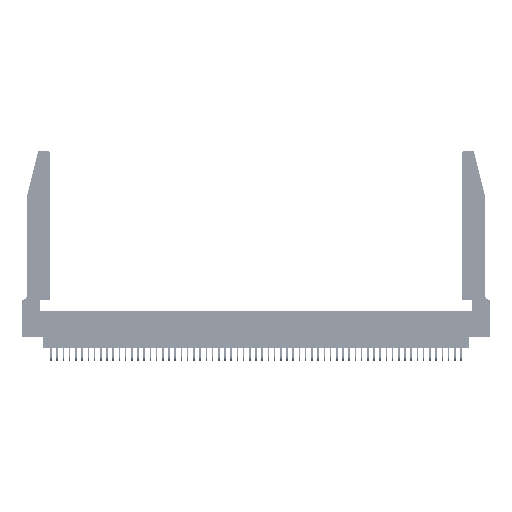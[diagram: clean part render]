
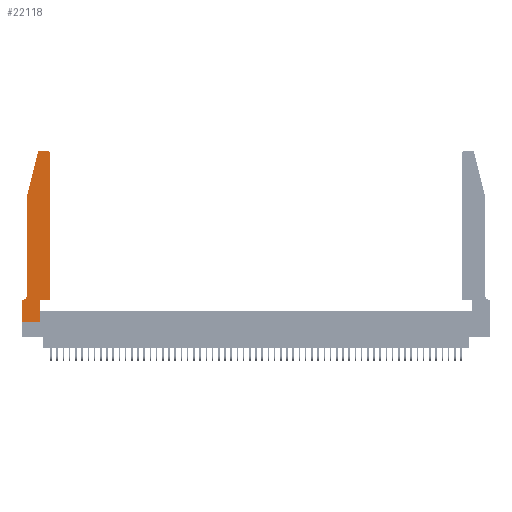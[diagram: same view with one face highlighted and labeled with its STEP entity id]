
A CAD part, top view. The second image highlights one B-rep face of the part: STEP entity #22118.
In plain terms, the highlighted planar face has unit normal (0, 0, 1).
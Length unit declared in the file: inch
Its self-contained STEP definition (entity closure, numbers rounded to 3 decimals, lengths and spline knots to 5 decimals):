
#448 = CIRCLE ( 'NONE', #9576, 0.03 ) ;
#577 = CARTESIAN_POINT ( 'NONE',  ( 0.4505, 0.35, 0.37 ) ) ;
#1251 = VERTEX_POINT ( 'NONE', #31348 ) ;
#1568 = LINE ( 'NONE', #27744, #34705 ) ;
#2363 = CARTESIAN_POINT ( 'NONE',  ( 0., 0.35, 0.37 ) ) ;
#2644 = ORIENTED_EDGE ( 'NONE', *, *, #7055, .T. ) ;
#3427 = VECTOR ( 'NONE', #39457, 39.37008 ) ;
#4058 = VERTEX_POINT ( 'NONE', #46979 ) ;
#4506 = VERTEX_POINT ( 'NONE', #54104 ) ;
#5450 = PLANE ( 'NONE',  #37151 ) ;
#6141 = DIRECTION ( 'NONE',  ( 0., -1., 0. ) ) ;
#7055 = EDGE_CURVE ( 'NONE', #8284, #24418, #36979, .T. ) ;
#7409 = LINE ( 'NONE', #52292, #51784 ) ;
#7909 = VERTEX_POINT ( 'NONE', #47162 ) ;
#8218 = CARTESIAN_POINT ( 'NONE',  ( 0.2865, 0.35, 0.37 ) ) ;
#8284 = VERTEX_POINT ( 'NONE', #2363 ) ;
#8522 = VERTEX_POINT ( 'NONE', #8218 ) ;
#9533 = ORIENTED_EDGE ( 'NONE', *, *, #33790, .T. ) ;
#9576 = AXIS2_PLACEMENT_3D ( 'NONE', #47927, #22349, #52252 ) ;
#9901 = DIRECTION ( 'NONE',  ( 0., 0., 1. ) ) ;
#10131 = ORIENTED_EDGE ( 'NONE', *, *, #50428, .T. ) ;
#10449 = VECTOR ( 'NONE', #50273, 39.37008 ) ;
#11404 = DIRECTION ( 'NONE',  ( 0., -1., 0. ) ) ;
#12452 = DIRECTION ( 'NONE',  ( -1., 0., 0. ) ) ;
#13493 = DIRECTION ( 'NONE',  ( 0., 0., -1. ) ) ;
#13606 = ORIENTED_EDGE ( 'NONE', *, *, #24213, .T. ) ;
#14256 = DIRECTION ( 'NONE',  ( 0., 0., 1. ) ) ;
#14684 = DIRECTION ( 'NONE',  ( 0., 1., 0. ) ) ;
#15362 = EDGE_CURVE ( 'NONE', #4506, #8284, #31526, .T. ) ;
#16904 = VECTOR ( 'NONE', #51063, 39.37008 ) ;
#18411 = CIRCLE ( 'NONE', #40693, 0.03 ) ;
#19035 = VERTEX_POINT ( 'NONE', #51246 ) ;
#19907 = EDGE_CURVE ( 'NONE', #24418, #42838, #7409, .T. ) ;
#20412 = VECTOR ( 'NONE', #41550, 39.37008 ) ;
#21118 = EDGE_CURVE ( 'NONE', #42838, #8522, #46048, .T. ) ;
#21649 = ORIENTED_EDGE ( 'NONE', *, *, #15362, .T. ) ;
#22118 = ADVANCED_FACE ( 'NONE', ( #40603 ), #5450, .T. ) ;
#22349 = DIRECTION ( 'NONE',  ( 0., 0., 1. ) ) ;
#22935 = EDGE_CURVE ( 'NONE', #7909, #19035, #44513, .T. ) ;
#24213 = EDGE_CURVE ( 'NONE', #54531, #1251, #48345, .T. ) ;
#24418 = VERTEX_POINT ( 'NONE', #31094 ) ;
#24508 = CARTESIAN_POINT ( 'NONE',  ( 0.0755, 2., 0.37 ) ) ;
#25098 = ORIENTED_EDGE ( 'NONE', *, *, #39977, .T. ) ;
#25170 = LINE ( 'NONE', #36088, #35232 ) ;
#26970 = VECTOR ( 'NONE', #11404, 39.37008 ) ;
#27744 = CARTESIAN_POINT ( 'NONE',  ( 0.0755, 2., 0.37 ) ) ;
#29682 = CARTESIAN_POINT ( 'NONE',  ( 0.4505, 2.72, 0.37 ) ) ;
#31094 = CARTESIAN_POINT ( 'NONE',  ( 0., 0., 0.37 ) ) ;
#31348 = CARTESIAN_POINT ( 'NONE',  ( 0.284, 2.75, 0.37 ) ) ;
#31526 = LINE ( 'NONE', #33915, #52906 ) ;
#31630 = EDGE_CURVE ( 'NONE', #1251, #7909, #18411, .T. ) ;
#33123 = ORIENTED_EDGE ( 'NONE', *, *, #54896, .T. ) ;
#33149 = CARTESIAN_POINT ( 'NONE',  ( 0.4205, 2.75, 0.37 ) ) ;
#33790 = EDGE_CURVE ( 'NONE', #4058, #55615, #25170, .T. ) ;
#33915 = CARTESIAN_POINT ( 'NONE',  ( 0.0755, 0.35, 0.37 ) ) ;
#34705 = VECTOR ( 'NONE', #6141, 39.37008 ) ;
#35115 = ORIENTED_EDGE ( 'NONE', *, *, #19907, .T. ) ;
#35232 = VECTOR ( 'NONE', #14684, 39.37008 ) ;
#35706 = CARTESIAN_POINT ( 'NONE',  ( 0.284, 2.72, 0.37 ) ) ;
#36088 = CARTESIAN_POINT ( 'NONE',  ( 0.4505, 0.35, 0.37 ) ) ;
#36979 = LINE ( 'NONE', #37169, #26970 ) ;
#37151 = AXIS2_PLACEMENT_3D ( 'NONE', #39939, #14256, #44235 ) ;
#37169 = CARTESIAN_POINT ( 'NONE',  ( 0., 0., 0.37 ) ) ;
#37402 = CARTESIAN_POINT ( 'NONE',  ( 0.2865, 0.35, 0.37 ) ) ;
#37843 = LINE ( 'NONE', #577, #3427 ) ;
#38003 = CARTESIAN_POINT ( 'NONE',  ( 0.2605, 2.75, 0.37 ) ) ;
#39045 = ORIENTED_EDGE ( 'NONE', *, *, #42927, .T. ) ;
#39201 = CARTESIAN_POINT ( 'NONE',  ( 0.0055, 0.42, 0.37 ) ) ;
#39457 = DIRECTION ( 'NONE',  ( 1., 0., 0. ) ) ;
#39591 = DIRECTION ( 'NONE',  ( 1., 0., 0. ) ) ;
#39700 = ORIENTED_EDGE ( 'NONE', *, *, #22935, .T. ) ;
#39939 = CARTESIAN_POINT ( 'NONE',  ( 0., 0.35, 0.37 ) ) ;
#39977 = EDGE_CURVE ( 'NONE', #55615, #54531, #448, .T. ) ;
#39990 = DIRECTION ( 'NONE',  ( 1., 0., 0. ) ) ;
#40065 = CARTESIAN_POINT ( 'NONE',  ( 0.2865, 0., 0.37 ) ) ;
#40451 = ORIENTED_EDGE ( 'NONE', *, *, #21118, .T. ) ;
#40603 = FACE_OUTER_BOUND ( 'NONE', #51782, .T. ) ;
#40693 = AXIS2_PLACEMENT_3D ( 'NONE', #35706, #9901, #39990 ) ;
#41550 = DIRECTION ( 'NONE',  ( -0.239, -0.971, 0. ) ) ;
#42838 = VERTEX_POINT ( 'NONE', #40065 ) ;
#42927 = EDGE_CURVE ( 'NONE', #19035, #50725, #1568, .T. ) ;
#43492 = DIRECTION ( 'NONE',  ( -1., 0., 0. ) ) ;
#43759 = CARTESIAN_POINT ( 'NONE',  ( 0.0755, 0.42, 0.37 ) ) ;
#44235 = DIRECTION ( 'NONE',  ( 1., 0., 0. ) ) ;
#44513 = LINE ( 'NONE', #24508, #20412 ) ;
#46048 = LINE ( 'NONE', #37402, #10449 ) ;
#46561 = AXIS2_PLACEMENT_3D ( 'NONE', #39201, #13493, #43492 ) ;
#46979 = CARTESIAN_POINT ( 'NONE',  ( 0.4505, 0.35, 0.37 ) ) ;
#47162 = CARTESIAN_POINT ( 'NONE',  ( 0.25487, 2.72718, 0.37 ) ) ;
#47770 = ORIENTED_EDGE ( 'NONE', *, *, #31630, .T. ) ;
#47927 = CARTESIAN_POINT ( 'NONE',  ( 0.4205, 2.72, 0.37 ) ) ;
#48345 = LINE ( 'NONE', #38003, #16904 ) ;
#48626 = CIRCLE ( 'NONE', #46561, 0.07 ) ;
#50273 = DIRECTION ( 'NONE',  ( 0., 1., 0. ) ) ;
#50428 = EDGE_CURVE ( 'NONE', #50725, #4506, #48626, .T. ) ;
#50725 = VERTEX_POINT ( 'NONE', #43759 ) ;
#51063 = DIRECTION ( 'NONE',  ( -1., 0., 0. ) ) ;
#51246 = CARTESIAN_POINT ( 'NONE',  ( 0.0755, 2., 0.37 ) ) ;
#51782 = EDGE_LOOP ( 'NONE', ( #13606, #47770, #39700, #39045, #10131, #21649, #2644, #35115, #40451, #33123, #9533, #25098 ) ) ;
#51784 = VECTOR ( 'NONE', #39591, 39.37008 ) ;
#52252 = DIRECTION ( 'NONE',  ( 1., 0., 0. ) ) ;
#52292 = CARTESIAN_POINT ( 'NONE',  ( 0., 0., 0.37 ) ) ;
#52906 = VECTOR ( 'NONE', #12452, 39.37008 ) ;
#54104 = CARTESIAN_POINT ( 'NONE',  ( 0.0055, 0.35, 0.37 ) ) ;
#54531 = VERTEX_POINT ( 'NONE', #33149 ) ;
#54896 = EDGE_CURVE ( 'NONE', #8522, #4058, #37843, .T. ) ;
#55615 = VERTEX_POINT ( 'NONE', #29682 ) ;
